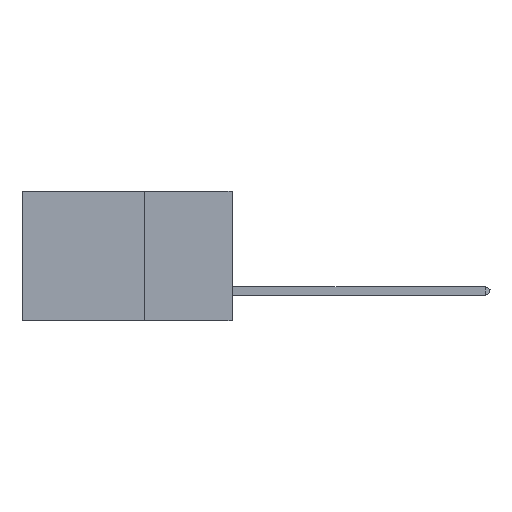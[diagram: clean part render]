
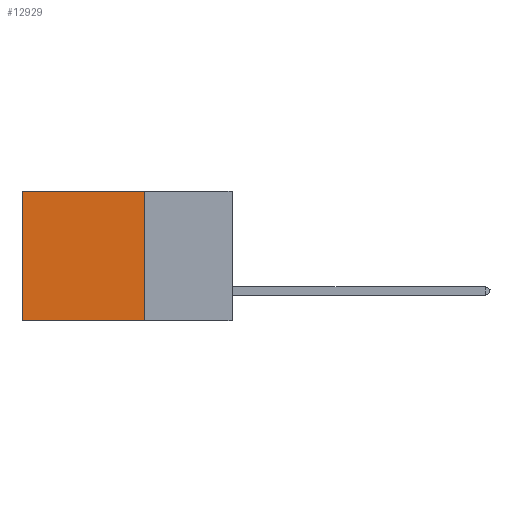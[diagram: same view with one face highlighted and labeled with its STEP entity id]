
A CAD part, left-side view. The second image highlights one B-rep face of the part: STEP entity #12929.
In plain terms, the highlighted planar face has unit normal (-1, 0, 0).
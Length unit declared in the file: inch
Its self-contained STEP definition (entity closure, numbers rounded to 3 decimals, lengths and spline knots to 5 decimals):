
#2347 = EDGE_CURVE ( 'NONE', #33047, #13230, #20719, .T. ) ;
#2468 = EDGE_CURVE ( 'NONE', #33047, #13004, #30533, .T. ) ;
#3144 = EDGE_CURVE ( 'NONE', #13004, #35878, #21122, .T. ) ;
#3591 = PLANE ( 'NONE',  #24916 ) ;
#4045 = DIRECTION ( 'NONE',  ( 0., 0., -1. ) ) ;
#4189 = CARTESIAN_POINT ( 'NONE',  ( 0.2875, 0.25, -0.37 ) ) ;
#5169 = VECTOR ( 'NONE', #18062, 39.37008 ) ;
#7168 = CARTESIAN_POINT ( 'NONE',  ( 0.2875, 0.25, 0. ) ) ;
#10191 = DIRECTION ( 'NONE',  ( 0., 1., 0. ) ) ;
#10358 = DIRECTION ( 'NONE',  ( 1., 0., 0. ) ) ;
#11986 = ORIENTED_EDGE ( 'NONE', *, *, #3144, .T. ) ;
#12929 = ADVANCED_FACE ( 'NONE', ( #22642 ), #3591, .F. ) ;
#13004 = VERTEX_POINT ( 'NONE', #25561 ) ;
#13230 = VERTEX_POINT ( 'NONE', #27853 ) ;
#15923 = CARTESIAN_POINT ( 'NONE',  ( 0.2875, 0.25, 0. ) ) ;
#18062 = DIRECTION ( 'NONE',  ( 0., 0., -1. ) ) ;
#19543 = ORIENTED_EDGE ( 'NONE', *, *, #2347, .F. ) ;
#20719 = LINE ( 'NONE', #27394, #23015 ) ;
#21122 = LINE ( 'NONE', #24336, #5169 ) ;
#22642 = FACE_OUTER_BOUND ( 'NONE', #23710, .T. ) ;
#23015 = VECTOR ( 'NONE', #4045, 39.37008 ) ;
#23710 = EDGE_LOOP ( 'NONE', ( #11986, #24420, #19543, #36070 ) ) ;
#24253 = EDGE_CURVE ( 'NONE', #13230, #35878, #34906, .T. ) ;
#24336 = CARTESIAN_POINT ( 'NONE',  ( 0.2875, 0.6, 0. ) ) ;
#24420 = ORIENTED_EDGE ( 'NONE', *, *, #24253, .F. ) ;
#24557 = CARTESIAN_POINT ( 'NONE',  ( 0.2875, 0.25, 0. ) ) ;
#24916 = AXIS2_PLACEMENT_3D ( 'NONE', #24557, #10358, #37404 ) ;
#25263 = DIRECTION ( 'NONE',  ( 0., 1., 0. ) ) ;
#25561 = CARTESIAN_POINT ( 'NONE',  ( 0.2875, 0.6, 0. ) ) ;
#27394 = CARTESIAN_POINT ( 'NONE',  ( 0.2875, 0.25, 0. ) ) ;
#27853 = CARTESIAN_POINT ( 'NONE',  ( 0.2875, 0.25, -0.37 ) ) ;
#30533 = LINE ( 'NONE', #7168, #35725 ) ;
#30667 = VECTOR ( 'NONE', #10191, 39.37008 ) ;
#31079 = CARTESIAN_POINT ( 'NONE',  ( 0.2875, 0.6, -0.37 ) ) ;
#33047 = VERTEX_POINT ( 'NONE', #15923 ) ;
#34906 = LINE ( 'NONE', #4189, #30667 ) ;
#35725 = VECTOR ( 'NONE', #25263, 39.37008 ) ;
#35878 = VERTEX_POINT ( 'NONE', #31079 ) ;
#36070 = ORIENTED_EDGE ( 'NONE', *, *, #2468, .T. ) ;
#37404 = DIRECTION ( 'NONE',  ( 0., 0., -1. ) ) ;
